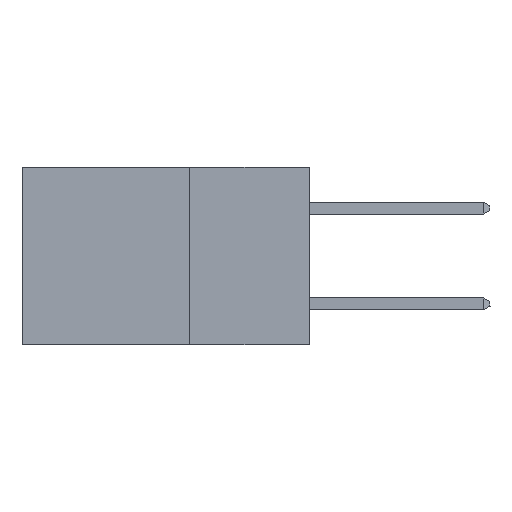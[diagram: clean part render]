
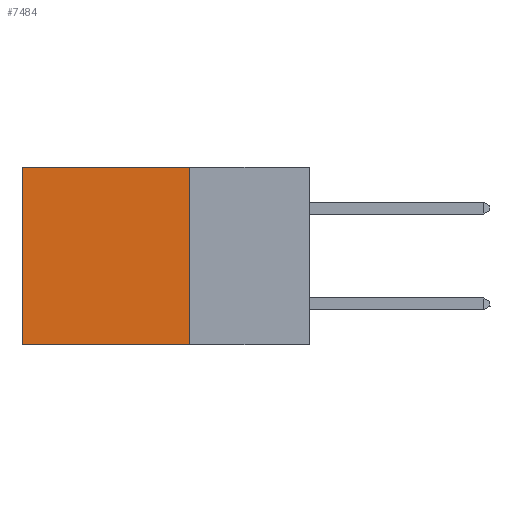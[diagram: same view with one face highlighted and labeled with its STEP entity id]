
A CAD part, left-side view. The second image highlights one B-rep face of the part: STEP entity #7484.
In plain terms, the highlighted planar face has unit normal (-1, 0, 0).
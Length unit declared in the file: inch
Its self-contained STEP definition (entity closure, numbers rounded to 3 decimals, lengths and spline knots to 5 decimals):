
#1668 = LINE ( 'NONE', #23982, #9530 ) ;
#2381 = DIRECTION ( 'NONE',  ( 0., 1., 0. ) ) ;
#2987 = PLANE ( 'NONE',  #8503 ) ;
#3934 = ORIENTED_EDGE ( 'NONE', *, *, #23995, .T. ) ;
#4581 = DIRECTION ( 'NONE',  ( 0., 1., 0. ) ) ;
#4598 = LINE ( 'NONE', #17531, #21669 ) ;
#4670 = VECTOR ( 'NONE', #4581, 39.37008 ) ;
#6576 = LINE ( 'NONE', #7497, #14479 ) ;
#6926 = EDGE_CURVE ( 'NONE', #18415, #7791, #4598, .T. ) ;
#7034 = ORIENTED_EDGE ( 'NONE', *, *, #6926, .T. ) ;
#7170 = ORIENTED_EDGE ( 'NONE', *, *, #18774, .F. ) ;
#7484 = ADVANCED_FACE ( 'NONE', ( #17630 ), #2987, .F. ) ;
#7497 = CARTESIAN_POINT ( 'NONE',  ( 0.2875, 0.25, 0. ) ) ;
#7791 = VERTEX_POINT ( 'NONE', #9745 ) ;
#8307 = CARTESIAN_POINT ( 'NONE',  ( 0.2875, 0.25, 0. ) ) ;
#8480 = CARTESIAN_POINT ( 'NONE',  ( 0.2875, 0.25, 0. ) ) ;
#8503 = AXIS2_PLACEMENT_3D ( 'NONE', #16530, #10762, #18493 ) ;
#9530 = VECTOR ( 'NONE', #2381, 39.37008 ) ;
#9745 = CARTESIAN_POINT ( 'NONE',  ( 0.2875, 0.6, -0.37 ) ) ;
#10198 = ORIENTED_EDGE ( 'NONE', *, *, #17049, .F. ) ;
#10762 = DIRECTION ( 'NONE',  ( 1., 0., 0. ) ) ;
#13865 = DIRECTION ( 'NONE',  ( 0., 0., -1. ) ) ;
#14479 = VECTOR ( 'NONE', #17338, 39.37008 ) ;
#14678 = LINE ( 'NONE', #8480, #4670 ) ;
#15143 = CARTESIAN_POINT ( 'NONE',  ( 0.2875, 0.25, -0.37 ) ) ;
#16530 = CARTESIAN_POINT ( 'NONE',  ( 0.2875, 0.25, 0. ) ) ;
#17049 = EDGE_CURVE ( 'NONE', #18768, #21247, #6576, .T. ) ;
#17338 = DIRECTION ( 'NONE',  ( 0., 0., -1. ) ) ;
#17531 = CARTESIAN_POINT ( 'NONE',  ( 0.2875, 0.6, 0. ) ) ;
#17630 = FACE_OUTER_BOUND ( 'NONE', #21964, .T. ) ;
#18415 = VERTEX_POINT ( 'NONE', #19274 ) ;
#18493 = DIRECTION ( 'NONE',  ( 0., 0., -1. ) ) ;
#18768 = VERTEX_POINT ( 'NONE', #8307 ) ;
#18774 = EDGE_CURVE ( 'NONE', #21247, #7791, #1668, .T. ) ;
#19274 = CARTESIAN_POINT ( 'NONE',  ( 0.2875, 0.6, 0. ) ) ;
#21247 = VERTEX_POINT ( 'NONE', #15143 ) ;
#21669 = VECTOR ( 'NONE', #13865, 39.37008 ) ;
#21964 = EDGE_LOOP ( 'NONE', ( #7034, #7170, #10198, #3934 ) ) ;
#23982 = CARTESIAN_POINT ( 'NONE',  ( 0.2875, 0.25, -0.37 ) ) ;
#23995 = EDGE_CURVE ( 'NONE', #18768, #18415, #14678, .T. ) ;
